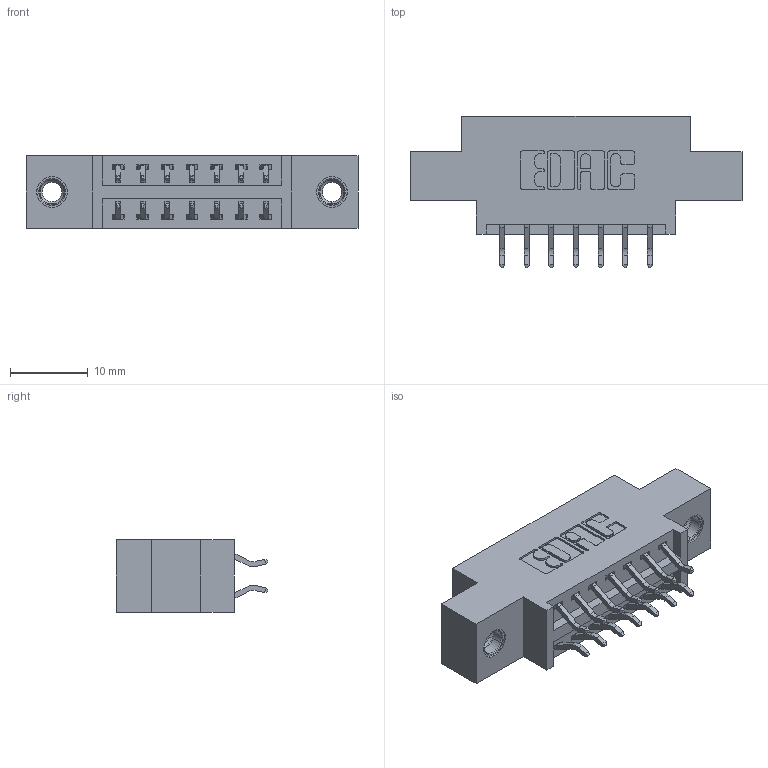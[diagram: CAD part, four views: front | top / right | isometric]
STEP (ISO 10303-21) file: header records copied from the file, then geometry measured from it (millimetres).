
FILE_DESCRIPTION (( 'STEP AP203' ), '1' );
FILE_NAME ('396-014-556-807.STEP', '2019-11-01T17:23:51', ( '' ), ( '' ), 'SwSTEP 2.0', 'SolidWorks 2016', '' );
FILE_SCHEMA (( 'CONFIG_CONTROL_DESIGN' ));
Length unit declared in the file: inch
Products named in the file (4): 345-250-001_345-250-005-103; 396-014-556-807; 346 Part_0.170 Offset - 0.156 Dia-TI; 345-292-001_556 Tail
Assembly tree (17 placements, depth 2):
  396-014-556-807
    346 Part_0.170 Offset - 0.156 Dia-TI
    345-292-001_556 Tail  x14
    345-250-001_345-250-005-103  x2
Bounding box: 42.8 x 19.57 x 9.4 mm (x, y, z)
Volume: 3732.9 mm3; surface area: 4781.4 mm2
Topology: 17 solids, 17 shells, 998 faces, 2899 edges, 1906 vertices
Faces by surface type: plane 658, cylinder 324, cone 12, torus 4
Entity records: 10818 total; most frequent: CARTESIAN_POINT 1831, ORIENTED_EDGE 1746, DIRECTION 1679, EDGE_CURVE 873, VECTOR 685, LINE 685, VERTEX_POINT 576, AXIS2_PLACEMENT_3D 497
